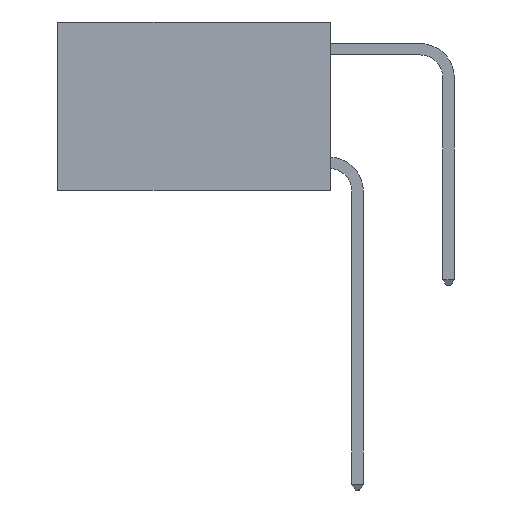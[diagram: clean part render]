
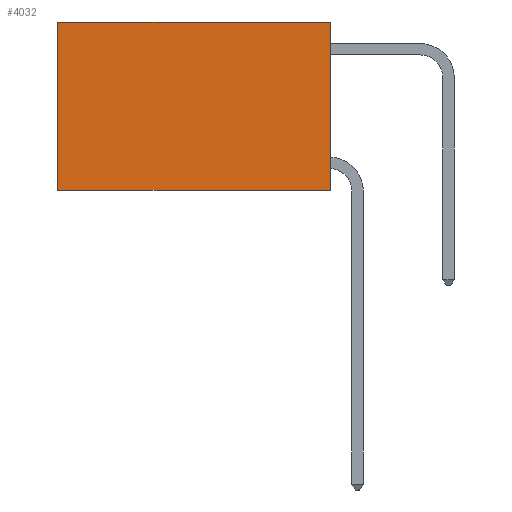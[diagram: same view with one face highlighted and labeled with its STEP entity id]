
A CAD part, left-side view. The second image highlights one B-rep face of the part: STEP entity #4032.
In plain terms, the highlighted planar face has unit normal (-1, 0, 0).
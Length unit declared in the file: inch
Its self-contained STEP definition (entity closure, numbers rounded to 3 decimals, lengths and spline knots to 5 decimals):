
#1107 = DIRECTION ( 'NONE',  ( 0., 0., -1. ) ) ;
#1115 = CARTESIAN_POINT ( 'NONE',  ( 0.2625, 0., 0. ) ) ;
#1240 = LINE ( 'NONE', #5729, #3614 ) ;
#1333 = CARTESIAN_POINT ( 'NONE',  ( 0.2625, 0.6, 0. ) ) ;
#1799 = DIRECTION ( 'NONE',  ( 0., 0., -1. ) ) ;
#1844 = CARTESIAN_POINT ( 'NONE',  ( 0.2625, 0.6, 0. ) ) ;
#1939 = ORIENTED_EDGE ( 'NONE', *, *, #8348, .F. ) ;
#2106 = VERTEX_POINT ( 'NONE', #1333 ) ;
#2340 = VECTOR ( 'NONE', #4744, 39.37008 ) ;
#2669 = EDGE_CURVE ( 'NONE', #5189, #2106, #1240, .T. ) ;
#2739 = CARTESIAN_POINT ( 'NONE',  ( 0.2625, 0., -0.37 ) ) ;
#2746 = ORIENTED_EDGE ( 'NONE', *, *, #3830, .F. ) ;
#2755 = LINE ( 'NONE', #1844, #8363 ) ;
#2789 = EDGE_CURVE ( 'NONE', #2106, #3467, #2755, .T. ) ;
#3467 = VERTEX_POINT ( 'NONE', #5500 ) ;
#3614 = VECTOR ( 'NONE', #5653, 39.37008 ) ;
#3816 = CARTESIAN_POINT ( 'NONE',  ( 0.2625, 0., -0.37 ) ) ;
#3830 = EDGE_CURVE ( 'NONE', #5189, #5863, #6033, .T. ) ;
#3860 = CARTESIAN_POINT ( 'NONE',  ( 0.2625, 0., 0. ) ) ;
#4032 = ADVANCED_FACE ( 'NONE', ( #6265 ), #9537, .F. ) ;
#4744 = DIRECTION ( 'NONE',  ( 0., 1., 0. ) ) ;
#5189 = VERTEX_POINT ( 'NONE', #3860 ) ;
#5429 = VECTOR ( 'NONE', #1107, 39.37008 ) ;
#5500 = CARTESIAN_POINT ( 'NONE',  ( 0.2625, 0.6, -0.37 ) ) ;
#5653 = DIRECTION ( 'NONE',  ( 0., 1., 0. ) ) ;
#5729 = CARTESIAN_POINT ( 'NONE',  ( 0.2625, 0., 0. ) ) ;
#5863 = VERTEX_POINT ( 'NONE', #2739 ) ;
#6033 = LINE ( 'NONE', #1115, #5429 ) ;
#6192 = LINE ( 'NONE', #3816, #2340 ) ;
#6265 = FACE_OUTER_BOUND ( 'NONE', #7875, .T. ) ;
#7057 = ORIENTED_EDGE ( 'NONE', *, *, #2789, .T. ) ;
#7875 = EDGE_LOOP ( 'NONE', ( #7057, #1939, #2746, #9705 ) ) ;
#8348 = EDGE_CURVE ( 'NONE', #5863, #3467, #6192, .T. ) ;
#8363 = VECTOR ( 'NONE', #1799, 39.37008 ) ;
#9214 = AXIS2_PLACEMENT_3D ( 'NONE', #9527, #9513, #9500 ) ;
#9500 = DIRECTION ( 'NONE',  ( 0., 0., -1. ) ) ;
#9513 = DIRECTION ( 'NONE',  ( 1., 0., 0. ) ) ;
#9527 = CARTESIAN_POINT ( 'NONE',  ( 0.2625, 0., 0. ) ) ;
#9537 = PLANE ( 'NONE',  #9214 ) ;
#9705 = ORIENTED_EDGE ( 'NONE', *, *, #2669, .T. ) ;
